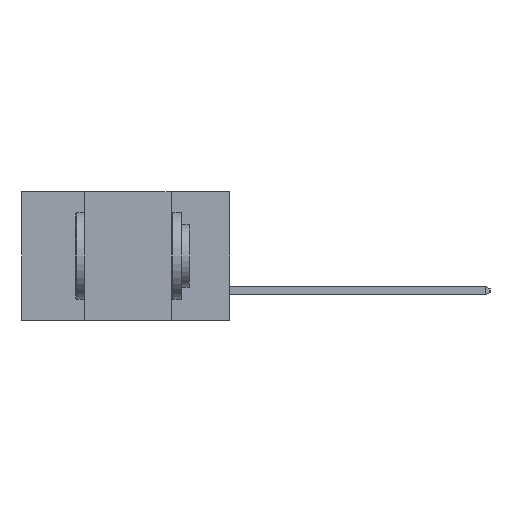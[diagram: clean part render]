
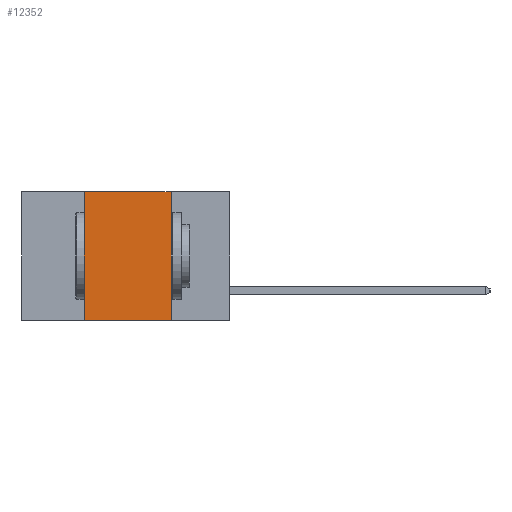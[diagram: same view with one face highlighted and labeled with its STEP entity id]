
A CAD part, left-side view. The second image highlights one B-rep face of the part: STEP entity #12352.
In plain terms, the highlighted planar face has unit normal (-1, 0, 0).
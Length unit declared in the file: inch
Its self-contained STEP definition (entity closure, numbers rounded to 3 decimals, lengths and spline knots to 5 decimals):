
#51 = EDGE_LOOP ( 'NONE', ( #18909, #15322, #20329, #8986 ) ) ;
#359 = DIRECTION ( 'NONE',  ( 0., 0., -1. ) ) ;
#605 = VERTEX_POINT ( 'NONE', #5294 ) ;
#1647 = DIRECTION ( 'NONE',  ( 1., 0., 0. ) ) ;
#1674 = PLANE ( 'NONE',  #10109 ) ;
#2527 = LINE ( 'NONE', #6856, #10531 ) ;
#2956 = VERTEX_POINT ( 'NONE', #11588 ) ;
#3741 = DIRECTION ( 'NONE',  ( 0., 0., 1. ) ) ;
#4783 = CARTESIAN_POINT ( 'NONE',  ( 0., 0.6, 0. ) ) ;
#4963 = VERTEX_POINT ( 'NONE', #18806 ) ;
#5294 = CARTESIAN_POINT ( 'NONE',  ( 0., 0.42, 0. ) ) ;
#6392 = CARTESIAN_POINT ( 'NONE',  ( 0., 0.6, 0. ) ) ;
#6622 = CARTESIAN_POINT ( 'NONE',  ( 0., 0.6, -0.37 ) ) ;
#6856 = CARTESIAN_POINT ( 'NONE',  ( 0., 0.17, 0. ) ) ;
#7359 = VECTOR ( 'NONE', #3741, 39.37008 ) ;
#8015 = DIRECTION ( 'NONE',  ( 0., -1., 0. ) ) ;
#8986 = ORIENTED_EDGE ( 'NONE', *, *, #18297, .T. ) ;
#10109 = AXIS2_PLACEMENT_3D ( 'NONE', #4783, #1647, #12779 ) ;
#10531 = VECTOR ( 'NONE', #359, 39.37008 ) ;
#10866 = VECTOR ( 'NONE', #17533, 39.37008 ) ;
#11588 = CARTESIAN_POINT ( 'NONE',  ( 0., 0.42, -0.37 ) ) ;
#12352 = ADVANCED_FACE ( 'NONE', ( #19457 ), #1674, .F. ) ;
#12779 = DIRECTION ( 'NONE',  ( 0., 0., -1. ) ) ;
#13047 = EDGE_CURVE ( 'NONE', #605, #4963, #19668, .T. ) ;
#14974 = LINE ( 'NONE', #6622, #10866 ) ;
#15322 = ORIENTED_EDGE ( 'NONE', *, *, #13047, .F. ) ;
#15585 = VECTOR ( 'NONE', #8015, 39.37008 ) ;
#15659 = LINE ( 'NONE', #17798, #7359 ) ;
#17329 = CARTESIAN_POINT ( 'NONE',  ( 0., 0.17, -0.37 ) ) ;
#17533 = DIRECTION ( 'NONE',  ( 0., -1., 0. ) ) ;
#17798 = CARTESIAN_POINT ( 'NONE',  ( 0., 0.42, 0. ) ) ;
#18235 = VERTEX_POINT ( 'NONE', #17329 ) ;
#18297 = EDGE_CURVE ( 'NONE', #2956, #18235, #14974, .T. ) ;
#18806 = CARTESIAN_POINT ( 'NONE',  ( 0., 0.17, 0. ) ) ;
#18909 = ORIENTED_EDGE ( 'NONE', *, *, #20345, .F. ) ;
#19344 = EDGE_CURVE ( 'NONE', #2956, #605, #15659, .T. ) ;
#19457 = FACE_OUTER_BOUND ( 'NONE', #51, .T. ) ;
#19668 = LINE ( 'NONE', #6392, #15585 ) ;
#20329 = ORIENTED_EDGE ( 'NONE', *, *, #19344, .F. ) ;
#20345 = EDGE_CURVE ( 'NONE', #4963, #18235, #2527, .T. ) ;
